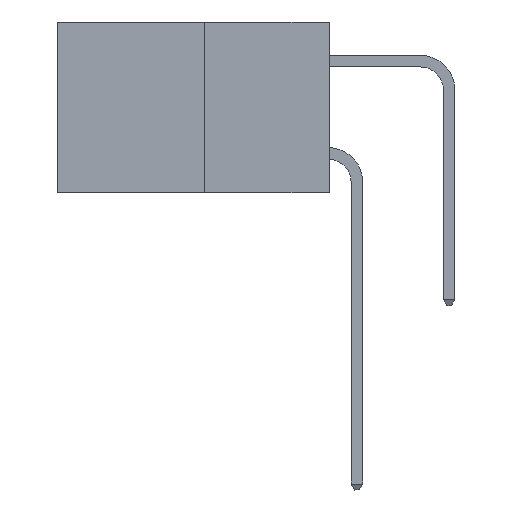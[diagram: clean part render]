
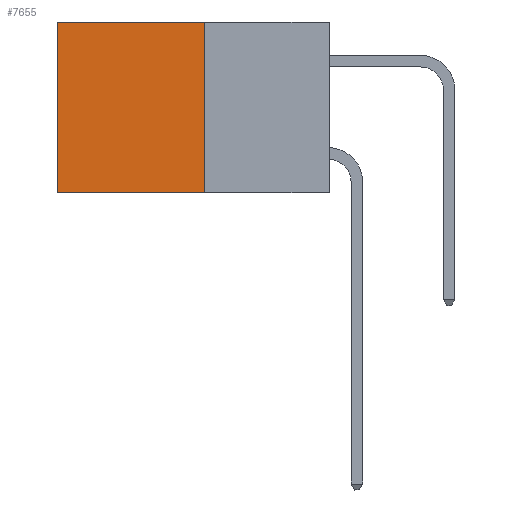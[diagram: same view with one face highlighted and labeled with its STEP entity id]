
A CAD part, left-side view. The second image highlights one B-rep face of the part: STEP entity #7655.
In plain terms, the highlighted planar face has unit normal (-1, 0, 0).
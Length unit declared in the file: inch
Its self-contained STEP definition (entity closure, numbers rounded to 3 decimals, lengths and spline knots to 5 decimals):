
#213 = EDGE_CURVE ( 'NONE', #23703, #12963, #15400, .T. ) ;
#373 = ORIENTED_EDGE ( 'NONE', *, *, #213, .T. ) ;
#451 = AXIS2_PLACEMENT_3D ( 'NONE', #8628, #21338, #10465 ) ;
#486 = ORIENTED_EDGE ( 'NONE', *, *, #3499, .T. ) ;
#1375 = CARTESIAN_POINT ( 'NONE',  ( 0.277, 0.59, -0.37 ) ) ;
#1500 = VECTOR ( 'NONE', #3458, 39.37008 ) ;
#1608 = EDGE_CURVE ( 'NONE', #1612, #12963, #20995, .T. ) ;
#1612 = VERTEX_POINT ( 'NONE', #12709 ) ;
#2476 = VECTOR ( 'NONE', #9477, 39.37008 ) ;
#3458 = DIRECTION ( 'NONE',  ( 0., 1., 0. ) ) ;
#3499 = EDGE_CURVE ( 'NONE', #21928, #23703, #5536, .T. ) ;
#4939 = CARTESIAN_POINT ( 'NONE',  ( 0.277, 0.27, 0. ) ) ;
#5536 = LINE ( 'NONE', #4939, #10425 ) ;
#7621 = CARTESIAN_POINT ( 'NONE',  ( 0.277, 0.27, -0.37 ) ) ;
#7655 = ADVANCED_FACE ( 'NONE', ( #16072 ), #17710, .F. ) ;
#8628 = CARTESIAN_POINT ( 'NONE',  ( 0.277, 0.27, -0.37 ) ) ;
#9337 = CARTESIAN_POINT ( 'NONE',  ( 0.277, 0.59, -0.37 ) ) ;
#9477 = DIRECTION ( 'NONE',  ( 0., 0., -1. ) ) ;
#10425 = VECTOR ( 'NONE', #17726, 39.37008 ) ;
#10465 = DIRECTION ( 'NONE',  ( 0., 0., -1. ) ) ;
#10848 = DIRECTION ( 'NONE',  ( 0., 0., -1. ) ) ;
#12415 = EDGE_LOOP ( 'NONE', ( #373, #14806, #13859, #486 ) ) ;
#12709 = CARTESIAN_POINT ( 'NONE',  ( 0.277, 0.27, -0.37 ) ) ;
#12963 = VERTEX_POINT ( 'NONE', #1375 ) ;
#13428 = CARTESIAN_POINT ( 'NONE',  ( 0.277, 0.27, 0. ) ) ;
#13859 = ORIENTED_EDGE ( 'NONE', *, *, #21109, .F. ) ;
#14806 = ORIENTED_EDGE ( 'NONE', *, *, #1608, .F. ) ;
#14814 = VECTOR ( 'NONE', #10848, 39.37008 ) ;
#15400 = LINE ( 'NONE', #9337, #14814 ) ;
#15902 = CARTESIAN_POINT ( 'NONE',  ( 0.277, 0.59, 0. ) ) ;
#15976 = LINE ( 'NONE', #7621, #2476 ) ;
#16072 = FACE_OUTER_BOUND ( 'NONE', #12415, .T. ) ;
#17710 = PLANE ( 'NONE',  #451 ) ;
#17726 = DIRECTION ( 'NONE',  ( 0., 1., 0. ) ) ;
#20995 = LINE ( 'NONE', #21662, #1500 ) ;
#21109 = EDGE_CURVE ( 'NONE', #21928, #1612, #15976, .T. ) ;
#21338 = DIRECTION ( 'NONE',  ( 1., 0., 0. ) ) ;
#21662 = CARTESIAN_POINT ( 'NONE',  ( 0.277, 0.27, -0.37 ) ) ;
#21928 = VERTEX_POINT ( 'NONE', #13428 ) ;
#23703 = VERTEX_POINT ( 'NONE', #15902 ) ;
